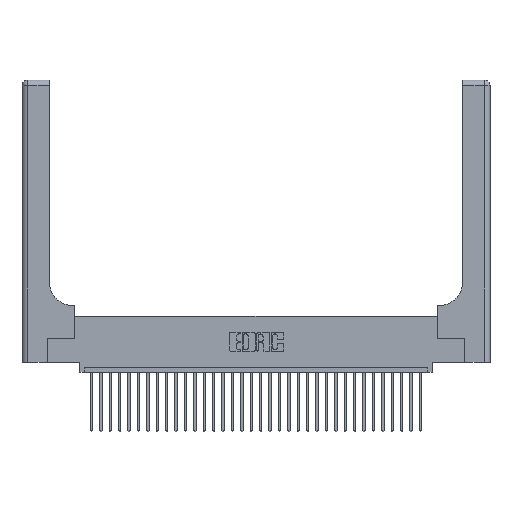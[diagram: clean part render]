
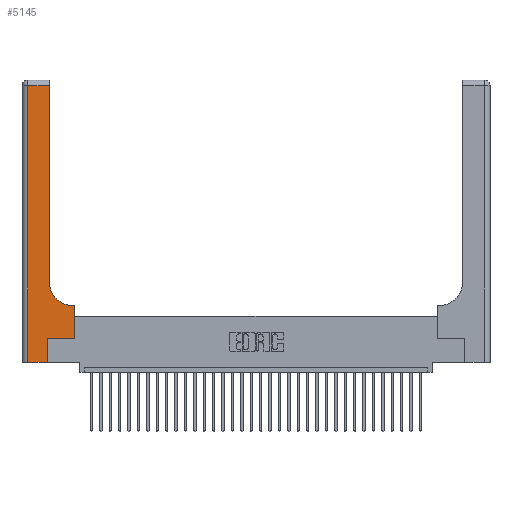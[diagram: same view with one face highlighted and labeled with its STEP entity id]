
A CAD part, top view. The second image highlights one B-rep face of the part: STEP entity #5145.
In plain terms, the highlighted planar face has unit normal (0, 0, 1).
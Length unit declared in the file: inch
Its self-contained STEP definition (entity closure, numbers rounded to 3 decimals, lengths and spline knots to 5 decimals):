
#312 = DIRECTION ( 'NONE',  ( 0., 0., -1. ) ) ;
#927 = DIRECTION ( 'NONE',  ( 0., 1., 0. ) ) ;
#1939 = CARTESIAN_POINT ( 'NONE',  ( 0.5585, 0.25, 0.37 ) ) ;
#2446 = EDGE_CURVE ( 'NONE', #31023, #28587, #29095, .T. ) ;
#3549 = CARTESIAN_POINT ( 'NONE',  ( 0.06, 0., 0.37 ) ) ;
#3858 = CARTESIAN_POINT ( 'NONE',  ( 0.2915, 0.85, 0.37 ) ) ;
#4063 = VECTOR ( 'NONE', #5684, 39.37008 ) ;
#4309 = VERTEX_POINT ( 'NONE', #30299 ) ;
#4678 = ORIENTED_EDGE ( 'NONE', *, *, #28802, .T. ) ;
#4940 = DIRECTION ( 'NONE',  ( 1., 0., 0. ) ) ;
#5145 = ADVANCED_FACE ( 'NONE', ( #14840 ), #21688, .F. ) ;
#5488 = CARTESIAN_POINT ( 'NONE',  ( 0.5415, 0.6, 0.37 ) ) ;
#5684 = DIRECTION ( 'NONE',  ( 0., 1., 0. ) ) ;
#8147 = CARTESIAN_POINT ( 'NONE',  ( 0., 0., 0.37 ) ) ;
#8294 = EDGE_CURVE ( 'NONE', #4309, #31023, #16990, .T. ) ;
#9660 = LINE ( 'NONE', #21063, #4063 ) ;
#10542 = CARTESIAN_POINT ( 'NONE',  ( 0.2915, 3., 0.37 ) ) ;
#10759 = ORIENTED_EDGE ( 'NONE', *, *, #26133, .T. ) ;
#11564 = LINE ( 'NONE', #32779, #26391 ) ;
#12374 = CIRCLE ( 'NONE', #21819, 0.25 ) ;
#12592 = ORIENTED_EDGE ( 'NONE', *, *, #23928, .T. ) ;
#12643 = DIRECTION ( 'NONE',  ( -1., 0., 0. ) ) ;
#13615 = DIRECTION ( 'NONE',  ( 0., 0., -1. ) ) ;
#14496 = CARTESIAN_POINT ( 'NONE',  ( 0., 2.94, 0.37 ) ) ;
#14840 = FACE_OUTER_BOUND ( 'NONE', #29636, .T. ) ;
#14972 = AXIS2_PLACEMENT_3D ( 'NONE', #18822, #13615, #21579 ) ;
#15006 = VERTEX_POINT ( 'NONE', #17597 ) ;
#15351 = CARTESIAN_POINT ( 'NONE',  ( 0.5415, 0.85, 0.37 ) ) ;
#15478 = EDGE_CURVE ( 'NONE', #28587, #15951, #29801, .T. ) ;
#15658 = ORIENTED_EDGE ( 'NONE', *, *, #2446, .T. ) ;
#15887 = EDGE_CURVE ( 'NONE', #17125, #4309, #24529, .T. ) ;
#15951 = VERTEX_POINT ( 'NONE', #18861 ) ;
#16114 = CARTESIAN_POINT ( 'NONE',  ( 0.06, 3., 0.37 ) ) ;
#16713 = CARTESIAN_POINT ( 'NONE',  ( 0.269, 0., 0.37 ) ) ;
#16990 = LINE ( 'NONE', #14496, #24211 ) ;
#17125 = VERTEX_POINT ( 'NONE', #3858 ) ;
#17597 = CARTESIAN_POINT ( 'NONE',  ( 0.5585, 0.6, 0.37 ) ) ;
#17702 = VECTOR ( 'NONE', #28483, 39.37008 ) ;
#17822 = CARTESIAN_POINT ( 'NONE',  ( 0.2915, 0.6, 0.37 ) ) ;
#18822 = CARTESIAN_POINT ( 'NONE',  ( 0., 3., 0.37 ) ) ;
#18861 = CARTESIAN_POINT ( 'NONE',  ( 0.269, 0., 0.37 ) ) ;
#19349 = CARTESIAN_POINT ( 'NONE',  ( 0.06, 2.94, 0.37 ) ) ;
#19670 = VERTEX_POINT ( 'NONE', #30502 ) ;
#19979 = DIRECTION ( 'NONE',  ( -1., 0., 0. ) ) ;
#20054 = ORIENTED_EDGE ( 'NONE', *, *, #8294, .T. ) ;
#20181 = ORIENTED_EDGE ( 'NONE', *, *, #15478, .T. ) ;
#21063 = CARTESIAN_POINT ( 'NONE',  ( 0.5585, 0.25, 0.37 ) ) ;
#21579 = DIRECTION ( 'NONE',  ( -1., 0., 0. ) ) ;
#21688 = PLANE ( 'NONE',  #14972 ) ;
#21819 = AXIS2_PLACEMENT_3D ( 'NONE', #15351, #312, #31041 ) ;
#22349 = ORIENTED_EDGE ( 'NONE', *, *, #31319, .T. ) ;
#22914 = EDGE_CURVE ( 'NONE', #15951, #19670, #28487, .T. ) ;
#23928 = EDGE_CURVE ( 'NONE', #27286, #17125, #12374, .T. ) ;
#24211 = VECTOR ( 'NONE', #19979, 39.37008 ) ;
#24529 = LINE ( 'NONE', #10542, #17702 ) ;
#25347 = VECTOR ( 'NONE', #28683, 39.37008 ) ;
#25378 = VERTEX_POINT ( 'NONE', #1939 ) ;
#26133 = EDGE_CURVE ( 'NONE', #25378, #15006, #9660, .T. ) ;
#26391 = VECTOR ( 'NONE', #4940, 39.37008 ) ;
#27286 = VERTEX_POINT ( 'NONE', #5488 ) ;
#28058 = VECTOR ( 'NONE', #927, 39.37008 ) ;
#28483 = DIRECTION ( 'NONE',  ( 0., 1., 0. ) ) ;
#28487 = LINE ( 'NONE', #16713, #28058 ) ;
#28587 = VERTEX_POINT ( 'NONE', #3549 ) ;
#28654 = VECTOR ( 'NONE', #29012, 39.37008 ) ;
#28683 = DIRECTION ( 'NONE',  ( 1., 0., 0. ) ) ;
#28802 = EDGE_CURVE ( 'NONE', #15006, #27286, #30190, .T. ) ;
#29012 = DIRECTION ( 'NONE',  ( 0., -1., 0. ) ) ;
#29095 = LINE ( 'NONE', #16114, #28654 ) ;
#29636 = EDGE_LOOP ( 'NONE', ( #30131, #20054, #15658, #20181, #31208, #22349, #10759, #4678, #12592 ) ) ;
#29801 = LINE ( 'NONE', #8147, #25347 ) ;
#30131 = ORIENTED_EDGE ( 'NONE', *, *, #15887, .T. ) ;
#30190 = LINE ( 'NONE', #17822, #30570 ) ;
#30299 = CARTESIAN_POINT ( 'NONE',  ( 0.2915, 2.94, 0.37 ) ) ;
#30502 = CARTESIAN_POINT ( 'NONE',  ( 0.269, 0.25, 0.37 ) ) ;
#30570 = VECTOR ( 'NONE', #12643, 39.37008 ) ;
#31023 = VERTEX_POINT ( 'NONE', #19349 ) ;
#31041 = DIRECTION ( 'NONE',  ( 1., 0., 0. ) ) ;
#31208 = ORIENTED_EDGE ( 'NONE', *, *, #22914, .T. ) ;
#31319 = EDGE_CURVE ( 'NONE', #19670, #25378, #11564, .T. ) ;
#32779 = CARTESIAN_POINT ( 'NONE',  ( 0.269, 0.25, 0.37 ) ) ;
